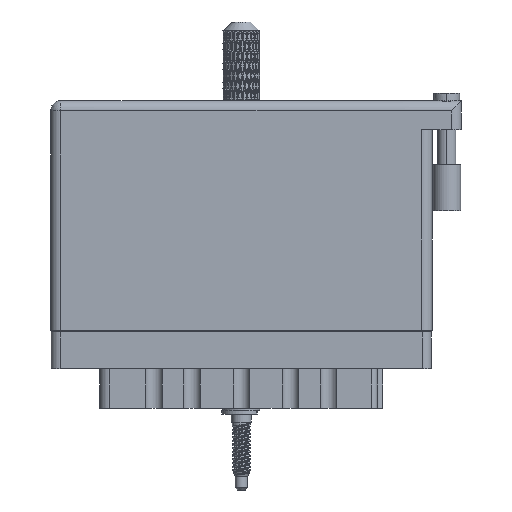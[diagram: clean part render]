
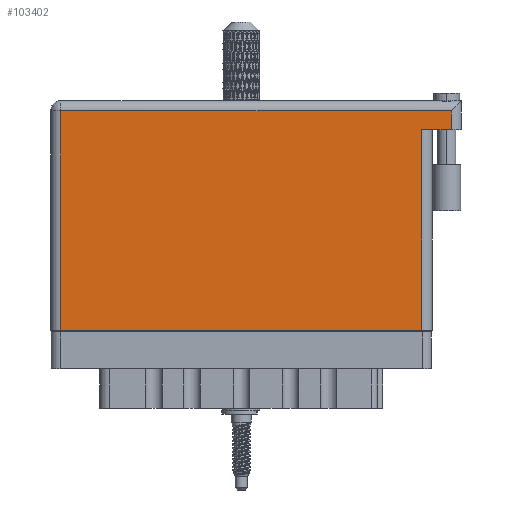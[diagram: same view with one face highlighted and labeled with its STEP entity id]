
A CAD part, front view. The second image highlights one B-rep face of the part: STEP entity #103402.
In plain terms, the highlighted face is planar.
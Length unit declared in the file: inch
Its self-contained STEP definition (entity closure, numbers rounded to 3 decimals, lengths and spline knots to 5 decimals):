
#574 = ORIENTED_EDGE ( 'NONE', *, *, #93294, .T. ) ;
#1385 = DIRECTION ( 'NONE',  ( 0., 1., 0. ) ) ;
#3380 = LINE ( 'NONE', #49390, #114024 ) ;
#6419 = VECTOR ( 'NONE', #119100, 39.37008 ) ;
#12118 = VERTEX_POINT ( 'NONE', #39071 ) ;
#12403 = ORIENTED_EDGE ( 'NONE', *, *, #81200, .T. ) ;
#14173 = EDGE_CURVE ( 'NONE', #72260, #12118, #3380, .T. ) ;
#20799 = CARTESIAN_POINT ( 'NONE',  ( 0.07, 0., 0. ) ) ;
#22575 = ORIENTED_EDGE ( 'NONE', *, *, #98991, .F. ) ;
#23269 = CARTESIAN_POINT ( 'NONE',  ( 0.07, 1.496, 0. ) ) ;
#25209 = CARTESIAN_POINT ( 'NONE',  ( 2.73, 1.369, 0. ) ) ;
#25593 = VECTOR ( 'NONE', #1385, 39.37008 ) ;
#25753 = CARTESIAN_POINT ( 'NONE',  ( 2.53, 0., 0. ) ) ;
#25871 = DIRECTION ( 'NONE',  ( -1., 0., 0. ) ) ;
#30886 = LINE ( 'NONE', #54814, #6419 ) ;
#35813 = LINE ( 'NONE', #80742, #57312 ) ;
#39071 = CARTESIAN_POINT ( 'NONE',  ( 2.73, 1.496, 0. ) ) ;
#49390 = CARTESIAN_POINT ( 'NONE',  ( 2.73, 1.566, 0. ) ) ;
#49909 = LINE ( 'NONE', #56399, #25593 ) ;
#51347 = DIRECTION ( 'NONE',  ( -1., 0., 0. ) ) ;
#51708 = ORIENTED_EDGE ( 'NONE', *, *, #14173, .T. ) ;
#51729 = DIRECTION ( 'NONE',  ( 0., 0., -1. ) ) ;
#52510 = PLANE ( 'NONE',  #94449 ) ;
#53715 = CARTESIAN_POINT ( 'NONE',  ( 0.07, 0., 0. ) ) ;
#54814 = CARTESIAN_POINT ( 'NONE',  ( 0., 0., 0. ) ) ;
#56399 = CARTESIAN_POINT ( 'NONE',  ( 2.53, 1.369, 0. ) ) ;
#56528 = DIRECTION ( 'NONE',  ( -1., 0., 0. ) ) ;
#57312 = VECTOR ( 'NONE', #25871, 39.37008 ) ;
#59406 = EDGE_CURVE ( 'NONE', #101845, #62418, #91937, .T. ) ;
#62418 = VERTEX_POINT ( 'NONE', #53715 ) ;
#69891 = VECTOR ( 'NONE', #56528, 39.37008 ) ;
#72260 = VERTEX_POINT ( 'NONE', #25209 ) ;
#78551 = EDGE_CURVE ( 'NONE', #90786, #102155, #49909, .T. ) ;
#80742 = CARTESIAN_POINT ( 'NONE',  ( 0., 1.496, 0. ) ) ;
#81200 = EDGE_CURVE ( 'NONE', #62418, #90786, #30886, .T. ) ;
#82954 = ORIENTED_EDGE ( 'NONE', *, *, #78551, .T. ) ;
#83176 = ORIENTED_EDGE ( 'NONE', *, *, #59406, .T. ) ;
#85603 = LINE ( 'NONE', #111554, #69891 ) ;
#87113 = DIRECTION ( 'NONE',  ( 0., 1., 0. ) ) ;
#90786 = VERTEX_POINT ( 'NONE', #25753 ) ;
#91937 = LINE ( 'NONE', #20799, #96194 ) ;
#93010 = CARTESIAN_POINT ( 'NONE',  ( 2.53, 1.369, 0. ) ) ;
#93294 = EDGE_CURVE ( 'NONE', #12118, #101845, #35813, .T. ) ;
#94449 = AXIS2_PLACEMENT_3D ( 'NONE', #116040, #51729, #51347 ) ;
#96194 = VECTOR ( 'NONE', #104640, 39.37008 ) ;
#98991 = EDGE_CURVE ( 'NONE', #72260, #102155, #85603, .T. ) ;
#101845 = VERTEX_POINT ( 'NONE', #23269 ) ;
#102155 = VERTEX_POINT ( 'NONE', #93010 ) ;
#103402 = ADVANCED_FACE ( 'NONE', ( #106544 ), #52510, .F. ) ;
#104640 = DIRECTION ( 'NONE',  ( 0., -1., 0. ) ) ;
#106544 = FACE_OUTER_BOUND ( 'NONE', #109650, .T. ) ;
#109650 = EDGE_LOOP ( 'NONE', ( #12403, #82954, #22575, #51708, #574, #83176 ) ) ;
#111554 = CARTESIAN_POINT ( 'NONE',  ( 2.8, 1.369, 0. ) ) ;
#114024 = VECTOR ( 'NONE', #87113, 39.37008 ) ;
#116040 = CARTESIAN_POINT ( 'NONE',  ( 0., 1.566, 0. ) ) ;
#119100 = DIRECTION ( 'NONE',  ( 1., 0., 0. ) ) ;
